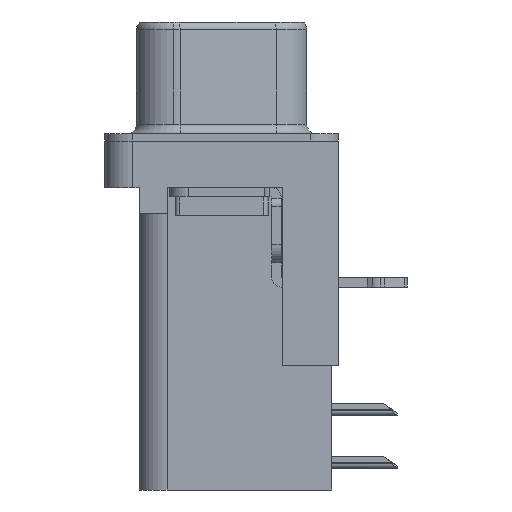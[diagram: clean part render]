
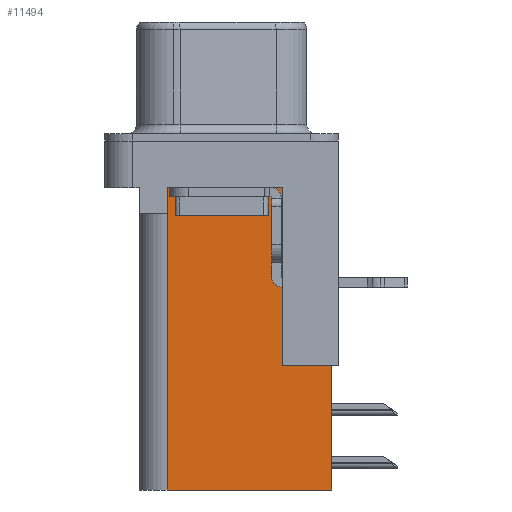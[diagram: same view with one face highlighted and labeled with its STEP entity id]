
A CAD part, left-side view. The second image highlights one B-rep face of the part: STEP entity #11494.
In plain terms, the highlighted planar face has unit normal (-1, 0, 0).
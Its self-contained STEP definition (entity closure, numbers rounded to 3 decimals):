
#53 = CARTESIAN_POINT ( 'NONE',  ( 3.7, -5.925, -18.76 ) ) ;
#212 = CARTESIAN_POINT ( 'NONE',  ( 3.7, 2.895, -2.5 ) ) ;
#463 = DIRECTION ( 'NONE',  ( 0., 0., 1. ) ) ;
#589 = ORIENTED_EDGE ( 'NONE', *, *, #17437, .T. ) ;
#1125 = CARTESIAN_POINT ( 'NONE',  ( 3.7, 2.925, -3.9 ) ) ;
#1286 = VECTOR ( 'NONE', #14236, 1000. ) ;
#1543 = FACE_OUTER_BOUND ( 'NONE', #12321, .T. ) ;
#1548 = LINE ( 'NONE', #5127, #2113 ) ;
#2077 = LINE ( 'NONE', #15274, #20477 ) ;
#2113 = VECTOR ( 'NONE', #6923, 1000. ) ;
#2983 = CARTESIAN_POINT ( 'NONE',  ( 3.7, 2.925, -18.76 ) ) ;
#3884 = LINE ( 'NONE', #5511, #8621 ) ;
#4506 = DIRECTION ( 'NONE',  ( 1., 0., 0. ) ) ;
#4685 = ORIENTED_EDGE ( 'NONE', *, *, #5375, .F. ) ;
#5127 = CARTESIAN_POINT ( 'NONE',  ( 3.7, -6.295, -12.05 ) ) ;
#5240 = VERTEX_POINT ( 'NONE', #2983 ) ;
#5375 = EDGE_CURVE ( 'NONE', #5240, #22260, #19510, .T. ) ;
#5511 = CARTESIAN_POINT ( 'NONE',  ( 3.7, -3.295, -18.76 ) ) ;
#5663 = EDGE_CURVE ( 'NONE', #19914, #12689, #18104, .T. ) ;
#6827 = CARTESIAN_POINT ( 'NONE',  ( 3.7, 2.895, -3.9 ) ) ;
#6898 = DIRECTION ( 'NONE',  ( 0., 0., 1. ) ) ;
#6923 = DIRECTION ( 'NONE',  ( 0., 1., 0. ) ) ;
#7159 = LINE ( 'NONE', #8840, #1286 ) ;
#7304 = DIRECTION ( 'NONE',  ( 0., 1., 0. ) ) ;
#7659 = EDGE_CURVE ( 'NONE', #14765, #22260, #7159, .T. ) ;
#8027 = VERTEX_POINT ( 'NONE', #11662 ) ;
#8621 = VECTOR ( 'NONE', #7304, 1000. ) ;
#8840 = CARTESIAN_POINT ( 'NONE',  ( 3.7, 0., -3.9 ) ) ;
#8906 = EDGE_CURVE ( 'NONE', #8027, #10560, #2077, .T. ) ;
#9019 = CARTESIAN_POINT ( 'NONE',  ( 3.7, -3.295, -12.05 ) ) ;
#9423 = ORIENTED_EDGE ( 'NONE', *, *, #8906, .F. ) ;
#10560 = VERTEX_POINT ( 'NONE', #53 ) ;
#10703 = ORIENTED_EDGE ( 'NONE', *, *, #5663, .T. ) ;
#10958 = CARTESIAN_POINT ( 'NONE',  ( 3.7, 2.895, -3.9 ) ) ;
#11494 = ADVANCED_FACE ( 'NONE', ( #1543 ), #15189, .F. ) ;
#11629 = CARTESIAN_POINT ( 'NONE',  ( 3.7, -3.295, -18.76 ) ) ;
#11662 = CARTESIAN_POINT ( 'NONE',  ( 3.7, -5.925, -12.05 ) ) ;
#11892 = VECTOR ( 'NONE', #17103, 1000. ) ;
#12193 = EDGE_CURVE ( 'NONE', #12689, #13713, #21322, .T. ) ;
#12321 = EDGE_LOOP ( 'NONE', ( #15991, #12914, #13874, #4685, #15855, #9423, #589, #10703 ) ) ;
#12689 = VERTEX_POINT ( 'NONE', #13065 ) ;
#12914 = ORIENTED_EDGE ( 'NONE', *, *, #18222, .T. ) ;
#13065 = CARTESIAN_POINT ( 'NONE',  ( 3.7, -3.295, -2.5 ) ) ;
#13713 = VERTEX_POINT ( 'NONE', #212 ) ;
#13874 = ORIENTED_EDGE ( 'NONE', *, *, #7659, .T. ) ;
#14236 = DIRECTION ( 'NONE',  ( 0., 1., 0. ) ) ;
#14765 = VERTEX_POINT ( 'NONE', #6827 ) ;
#14793 = VECTOR ( 'NONE', #6898, 1000. ) ;
#15189 = PLANE ( 'NONE',  #19345 ) ;
#15251 = VECTOR ( 'NONE', #16323, 1000. ) ;
#15274 = CARTESIAN_POINT ( 'NONE',  ( 3.7, -5.925, -2. ) ) ;
#15309 = CARTESIAN_POINT ( 'NONE',  ( 3.7, -3.295, -2.5 ) ) ;
#15855 = ORIENTED_EDGE ( 'NONE', *, *, #15911, .F. ) ;
#15911 = EDGE_CURVE ( 'NONE', #10560, #5240, #3884, .T. ) ;
#15991 = ORIENTED_EDGE ( 'NONE', *, *, #12193, .T. ) ;
#16323 = DIRECTION ( 'NONE',  ( 0., 0., -1. ) ) ;
#16985 = DIRECTION ( 'NONE',  ( 0., 1., 0. ) ) ;
#17103 = DIRECTION ( 'NONE',  ( 0., 1., 0. ) ) ;
#17437 = EDGE_CURVE ( 'NONE', #8027, #19914, #1548, .T. ) ;
#18104 = LINE ( 'NONE', #18258, #22242 ) ;
#18222 = EDGE_CURVE ( 'NONE', #13713, #14765, #19972, .T. ) ;
#18258 = CARTESIAN_POINT ( 'NONE',  ( 3.7, -3.295, -18.76 ) ) ;
#19345 = AXIS2_PLACEMENT_3D ( 'NONE', #11629, #4506, #16985 ) ;
#19510 = LINE ( 'NONE', #21066, #14793 ) ;
#19914 = VERTEX_POINT ( 'NONE', #9019 ) ;
#19972 = LINE ( 'NONE', #10958, #15251 ) ;
#20477 = VECTOR ( 'NONE', #20614, 1000. ) ;
#20614 = DIRECTION ( 'NONE',  ( 0., 0., -1. ) ) ;
#21066 = CARTESIAN_POINT ( 'NONE',  ( 3.7, 2.925, -18.76 ) ) ;
#21322 = LINE ( 'NONE', #15309, #11892 ) ;
#22242 = VECTOR ( 'NONE', #463, 1000. ) ;
#22260 = VERTEX_POINT ( 'NONE', #1125 ) ;
